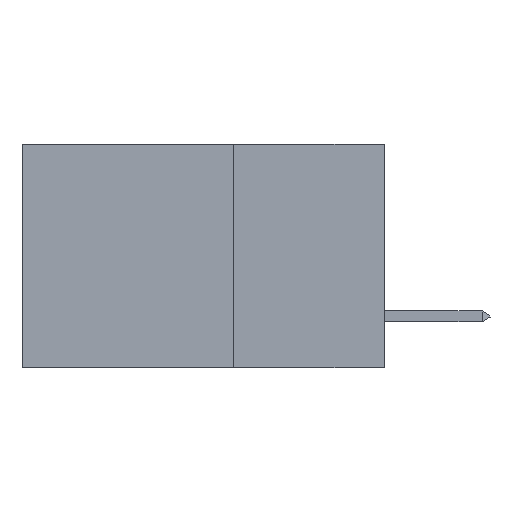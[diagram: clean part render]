
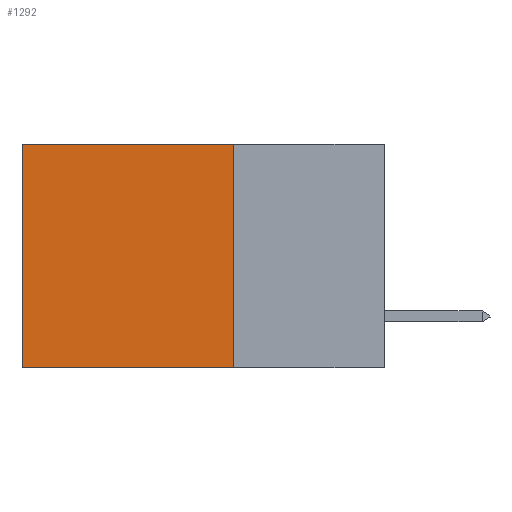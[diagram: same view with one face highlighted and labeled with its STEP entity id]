
A CAD part, left-side view. The second image highlights one B-rep face of the part: STEP entity #1292.
In plain terms, the highlighted planar face has unit normal (-1, 0, 0).
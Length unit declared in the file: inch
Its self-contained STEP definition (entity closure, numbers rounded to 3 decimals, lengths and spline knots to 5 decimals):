
#102 = DIRECTION ( 'NONE',  ( 0., 0., -1. ) ) ;
#227 = EDGE_CURVE ( 'NONE', #9898, #22413, #20802, .T. ) ;
#428 = PLANE ( 'NONE',  #12400 ) ;
#952 = LINE ( 'NONE', #4177, #20122 ) ;
#1248 = CARTESIAN_POINT ( 'NONE',  ( 0.2875, 0.25, 0. ) ) ;
#1292 = ADVANCED_FACE ( 'NONE', ( #28247 ), #428, .F. ) ;
#4177 = CARTESIAN_POINT ( 'NONE',  ( 0.2875, 0.25, -0.37 ) ) ;
#6066 = VECTOR ( 'NONE', #17441, 39.37008 ) ;
#6525 = EDGE_CURVE ( 'NONE', #15534, #21107, #15363, .T. ) ;
#6987 = CARTESIAN_POINT ( 'NONE',  ( 0.2875, 0.25, -0.37 ) ) ;
#9898 = VERTEX_POINT ( 'NONE', #23765 ) ;
#11864 = EDGE_CURVE ( 'NONE', #9898, #15534, #16534, .T. ) ;
#12400 = AXIS2_PLACEMENT_3D ( 'NONE', #18638, #18935, #27880 ) ;
#13123 = ORIENTED_EDGE ( 'NONE', *, *, #11864, .T. ) ;
#13728 = CARTESIAN_POINT ( 'NONE',  ( 0.2875, 0.6, -0.37 ) ) ;
#14368 = ORIENTED_EDGE ( 'NONE', *, *, #17127, .F. ) ;
#15363 = LINE ( 'NONE', #15513, #15709 ) ;
#15513 = CARTESIAN_POINT ( 'NONE',  ( 0.2875, 0.6, 0. ) ) ;
#15534 = VERTEX_POINT ( 'NONE', #29597 ) ;
#15709 = VECTOR ( 'NONE', #24758, 39.37008 ) ;
#16028 = EDGE_LOOP ( 'NONE', ( #27127, #14368, #20718, #13123 ) ) ;
#16534 = LINE ( 'NONE', #1248, #6066 ) ;
#17127 = EDGE_CURVE ( 'NONE', #22413, #21107, #952, .T. ) ;
#17441 = DIRECTION ( 'NONE',  ( 0., 1., 0. ) ) ;
#18638 = CARTESIAN_POINT ( 'NONE',  ( 0.2875, 0.25, 0. ) ) ;
#18935 = DIRECTION ( 'NONE',  ( 1., 0., 0. ) ) ;
#19746 = VECTOR ( 'NONE', #102, 39.37008 ) ;
#20122 = VECTOR ( 'NONE', #20318, 39.37008 ) ;
#20318 = DIRECTION ( 'NONE',  ( 0., 1., 0. ) ) ;
#20718 = ORIENTED_EDGE ( 'NONE', *, *, #227, .F. ) ;
#20802 = LINE ( 'NONE', #27769, #19746 ) ;
#21107 = VERTEX_POINT ( 'NONE', #13728 ) ;
#22413 = VERTEX_POINT ( 'NONE', #6987 ) ;
#23765 = CARTESIAN_POINT ( 'NONE',  ( 0.2875, 0.25, 0. ) ) ;
#24758 = DIRECTION ( 'NONE',  ( 0., 0., -1. ) ) ;
#27127 = ORIENTED_EDGE ( 'NONE', *, *, #6525, .T. ) ;
#27769 = CARTESIAN_POINT ( 'NONE',  ( 0.2875, 0.25, 0. ) ) ;
#27880 = DIRECTION ( 'NONE',  ( 0., 0., -1. ) ) ;
#28247 = FACE_OUTER_BOUND ( 'NONE', #16028, .T. ) ;
#29597 = CARTESIAN_POINT ( 'NONE',  ( 0.2875, 0.6, 0. ) ) ;
